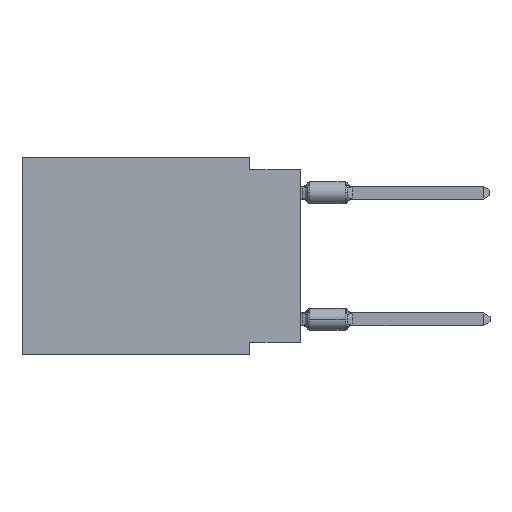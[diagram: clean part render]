
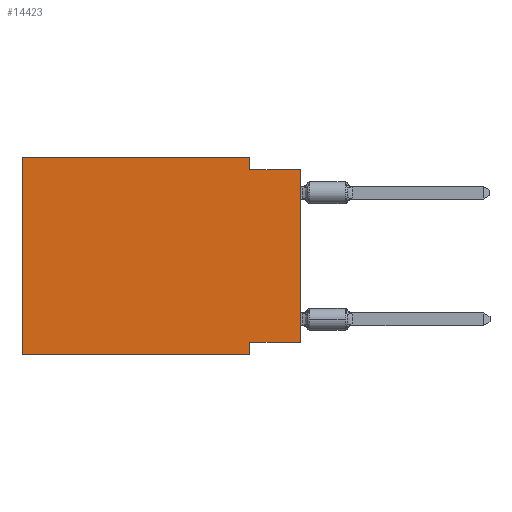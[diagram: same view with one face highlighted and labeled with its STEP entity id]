
A CAD part, left-side view. The second image highlights one B-rep face of the part: STEP entity #14423.
In plain terms, the highlighted planar face has unit normal (-1, 0, 0).
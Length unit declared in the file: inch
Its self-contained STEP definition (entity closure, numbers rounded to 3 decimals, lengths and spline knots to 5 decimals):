
#40 = EDGE_CURVE ( 'NONE', #4401, #25480, #16365, .T. ) ;
#192 = EDGE_CURVE ( 'NONE', #28392, #2258, #10923, .T. ) ;
#497 = CARTESIAN_POINT ( 'NONE',  ( 0., 0., 0. ) ) ;
#897 = CARTESIAN_POINT ( 'NONE',  ( 0., 0., -0.025 ) ) ;
#1308 = VERTEX_POINT ( 'NONE', #14144 ) ;
#1443 = CARTESIAN_POINT ( 'NONE',  ( 0., 0.55, 0. ) ) ;
#1731 = CARTESIAN_POINT ( 'NONE',  ( 0., 0., -0.365 ) ) ;
#1795 = CARTESIAN_POINT ( 'NONE',  ( 0., 0.1, -0.025 ) ) ;
#2258 = VERTEX_POINT ( 'NONE', #28420 ) ;
#2366 = DIRECTION ( 'NONE',  ( 0., 0., 1. ) ) ;
#2584 = LINE ( 'NONE', #897, #10356 ) ;
#2592 = EDGE_CURVE ( 'NONE', #6321, #1308, #24926, .T. ) ;
#2604 = CARTESIAN_POINT ( 'NONE',  ( 0., 0.1, 0. ) ) ;
#2760 = LINE ( 'NONE', #497, #21740 ) ;
#4401 = VERTEX_POINT ( 'NONE', #2604 ) ;
#4418 = DIRECTION ( 'NONE',  ( 0., 1., 0. ) ) ;
#4431 = DIRECTION ( 'NONE',  ( 0., 0., -1. ) ) ;
#4612 = LINE ( 'NONE', #9434, #20323 ) ;
#4629 = CARTESIAN_POINT ( 'NONE',  ( 0., 0., -0.025 ) ) ;
#4744 = LINE ( 'NONE', #25501, #26135 ) ;
#6321 = VERTEX_POINT ( 'NONE', #10060 ) ;
#6713 = DIRECTION ( 'NONE',  ( 0., -1., 0. ) ) ;
#7311 = ORIENTED_EDGE ( 'NONE', *, *, #8218, .F. ) ;
#8218 = EDGE_CURVE ( 'NONE', #29206, #4401, #8967, .T. ) ;
#8328 = AXIS2_PLACEMENT_3D ( 'NONE', #14546, #24166, #20245 ) ;
#8967 = LINE ( 'NONE', #27345, #25735 ) ;
#9221 = DIRECTION ( 'NONE',  ( 0., -1., 0. ) ) ;
#9434 = CARTESIAN_POINT ( 'NONE',  ( 0., 0.55, 0. ) ) ;
#9583 = CARTESIAN_POINT ( 'NONE',  ( 0., 0.1, 0. ) ) ;
#9976 = VECTOR ( 'NONE', #4418, 39.37008 ) ;
#10060 = CARTESIAN_POINT ( 'NONE',  ( 0., 0.55, -0.39 ) ) ;
#10356 = VECTOR ( 'NONE', #9221, 39.37008 ) ;
#10923 = LINE ( 'NONE', #1731, #9976 ) ;
#11231 = DIRECTION ( 'NONE',  ( 0., -1., 0. ) ) ;
#12219 = VECTOR ( 'NONE', #11231, 39.37008 ) ;
#12991 = ORIENTED_EDGE ( 'NONE', *, *, #14590, .F. ) ;
#13490 = CARTESIAN_POINT ( 'NONE',  ( 0., 0.55, -0.39 ) ) ;
#14144 = CARTESIAN_POINT ( 'NONE',  ( 0., 0.1, -0.39 ) ) ;
#14407 = FACE_OUTER_BOUND ( 'NONE', #26048, .T. ) ;
#14423 = ADVANCED_FACE ( 'NONE', ( #14407 ), #25989, .F. ) ;
#14546 = CARTESIAN_POINT ( 'NONE',  ( 0., 0.55, 0. ) ) ;
#14590 = EDGE_CURVE ( 'NONE', #2258, #1308, #4744, .T. ) ;
#14921 = ORIENTED_EDGE ( 'NONE', *, *, #192, .F. ) ;
#15492 = ORIENTED_EDGE ( 'NONE', *, *, #2592, .T. ) ;
#16365 = LINE ( 'NONE', #9583, #26376 ) ;
#16765 = ORIENTED_EDGE ( 'NONE', *, *, #23849, .T. ) ;
#17514 = CARTESIAN_POINT ( 'NONE',  ( 0., 0., -0.365 ) ) ;
#18589 = ORIENTED_EDGE ( 'NONE', *, *, #24524, .F. ) ;
#18860 = VERTEX_POINT ( 'NONE', #4629 ) ;
#20245 = DIRECTION ( 'NONE',  ( 0., 0., -1. ) ) ;
#20323 = VECTOR ( 'NONE', #2366, 39.37008 ) ;
#21740 = VECTOR ( 'NONE', #26071, 39.37008 ) ;
#23849 = EDGE_CURVE ( 'NONE', #28392, #18860, #2760, .T. ) ;
#24166 = DIRECTION ( 'NONE',  ( 1., 0., 0. ) ) ;
#24524 = EDGE_CURVE ( 'NONE', #6321, #29206, #4612, .T. ) ;
#24926 = LINE ( 'NONE', #13490, #12219 ) ;
#25480 = VERTEX_POINT ( 'NONE', #1795 ) ;
#25501 = CARTESIAN_POINT ( 'NONE',  ( 0., 0.1, -0.39 ) ) ;
#25682 = ORIENTED_EDGE ( 'NONE', *, *, #28668, .F. ) ;
#25735 = VECTOR ( 'NONE', #6713, 39.37008 ) ;
#25989 = PLANE ( 'NONE',  #8328 ) ;
#26048 = EDGE_LOOP ( 'NONE', ( #16765, #25682, #26841, #7311, #18589, #15492, #12991, #14921 ) ) ;
#26071 = DIRECTION ( 'NONE',  ( 0., 0., 1. ) ) ;
#26135 = VECTOR ( 'NONE', #4431, 39.37008 ) ;
#26376 = VECTOR ( 'NONE', #27659, 39.37008 ) ;
#26841 = ORIENTED_EDGE ( 'NONE', *, *, #40, .F. ) ;
#27345 = CARTESIAN_POINT ( 'NONE',  ( 0., 0.55, 0. ) ) ;
#27659 = DIRECTION ( 'NONE',  ( 0., 0., -1. ) ) ;
#28392 = VERTEX_POINT ( 'NONE', #17514 ) ;
#28420 = CARTESIAN_POINT ( 'NONE',  ( 0., 0.1, -0.365 ) ) ;
#28668 = EDGE_CURVE ( 'NONE', #25480, #18860, #2584, .T. ) ;
#29206 = VERTEX_POINT ( 'NONE', #1443 ) ;
